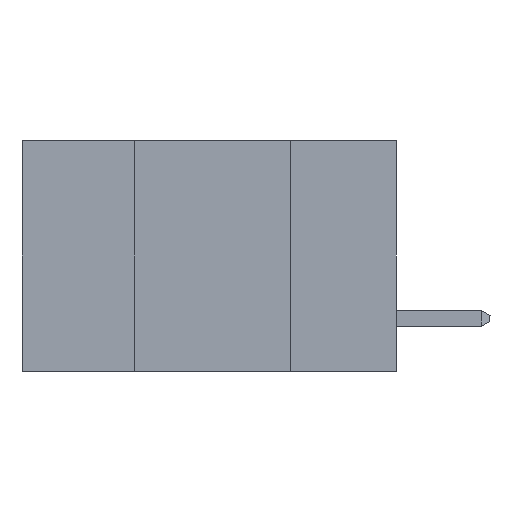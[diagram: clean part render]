
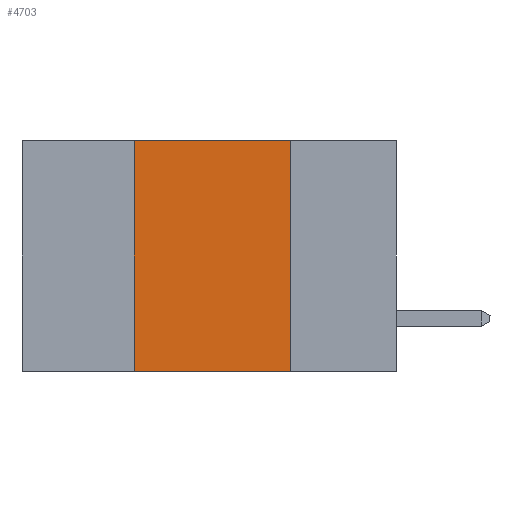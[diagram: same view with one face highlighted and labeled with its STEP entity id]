
A CAD part, left-side view. The second image highlights one B-rep face of the part: STEP entity #4703.
In plain terms, the highlighted planar face has unit normal (-1, 0, 0).
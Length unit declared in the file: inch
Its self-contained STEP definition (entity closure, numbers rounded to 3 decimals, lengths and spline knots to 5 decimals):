
#77 = CARTESIAN_POINT ( 'NONE',  ( 0., 0.17, -0.37 ) ) ;
#397 = VECTOR ( 'NONE', #15346, 39.37008 ) ;
#1214 = ORIENTED_EDGE ( 'NONE', *, *, #11624, .F. ) ;
#1672 = VECTOR ( 'NONE', #15471, 39.37008 ) ;
#2041 = EDGE_CURVE ( 'NONE', #15818, #3178, #12568, .T. ) ;
#2072 = ORIENTED_EDGE ( 'NONE', *, *, #2041, .F. ) ;
#2635 = CARTESIAN_POINT ( 'NONE',  ( 0., 0.42, -0.37 ) ) ;
#3031 = EDGE_CURVE ( 'NONE', #9057, #12324, #14123, .T. ) ;
#3178 = VERTEX_POINT ( 'NONE', #15878 ) ;
#3603 = FACE_OUTER_BOUND ( 'NONE', #13471, .T. ) ;
#4703 = ADVANCED_FACE ( 'NONE', ( #3603 ), #9843, .F. ) ;
#4838 = DIRECTION ( 'NONE',  ( 1., 0., 0. ) ) ;
#4842 = EDGE_CURVE ( 'NONE', #9057, #15818, #13550, .T. ) ;
#4916 = VECTOR ( 'NONE', #6532, 39.37008 ) ;
#5296 = CARTESIAN_POINT ( 'NONE',  ( 0., 0.6, 0. ) ) ;
#6182 = VECTOR ( 'NONE', #11110, 39.37008 ) ;
#6532 = DIRECTION ( 'NONE',  ( 0., 0., 1. ) ) ;
#6886 = DIRECTION ( 'NONE',  ( 0., 0., -1. ) ) ;
#8012 = CARTESIAN_POINT ( 'NONE',  ( 0., 0.42, 0. ) ) ;
#9057 = VERTEX_POINT ( 'NONE', #15709 ) ;
#9843 = PLANE ( 'NONE',  #13693 ) ;
#11047 = CARTESIAN_POINT ( 'NONE',  ( 0., 0.6, 0. ) ) ;
#11110 = DIRECTION ( 'NONE',  ( 0., -1., 0. ) ) ;
#11356 = ORIENTED_EDGE ( 'NONE', *, *, #3031, .T. ) ;
#11624 = EDGE_CURVE ( 'NONE', #3178, #12324, #13861, .T. ) ;
#11727 = CARTESIAN_POINT ( 'NONE',  ( 0., 0.17, -0.37 ) ) ;
#12324 = VERTEX_POINT ( 'NONE', #77 ) ;
#12568 = LINE ( 'NONE', #5296, #6182 ) ;
#13471 = EDGE_LOOP ( 'NONE', ( #1214, #2072, #15632, #11356 ) ) ;
#13550 = LINE ( 'NONE', #2635, #4916 ) ;
#13693 = AXIS2_PLACEMENT_3D ( 'NONE', #11047, #4838, #6886 ) ;
#13861 = LINE ( 'NONE', #11727, #397 ) ;
#14123 = LINE ( 'NONE', #15396, #1672 ) ;
#15346 = DIRECTION ( 'NONE',  ( 0., 0., -1. ) ) ;
#15396 = CARTESIAN_POINT ( 'NONE',  ( 0., 0.6, -0.37 ) ) ;
#15471 = DIRECTION ( 'NONE',  ( 0., -1., 0. ) ) ;
#15632 = ORIENTED_EDGE ( 'NONE', *, *, #4842, .F. ) ;
#15709 = CARTESIAN_POINT ( 'NONE',  ( 0., 0.42, -0.37 ) ) ;
#15818 = VERTEX_POINT ( 'NONE', #8012 ) ;
#15878 = CARTESIAN_POINT ( 'NONE',  ( 0., 0.17, 0. ) ) ;
